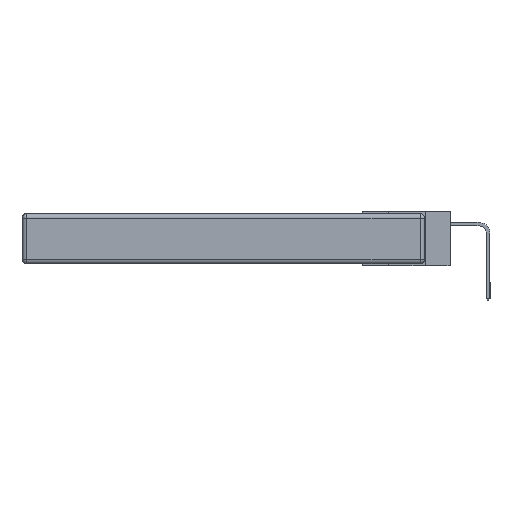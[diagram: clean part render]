
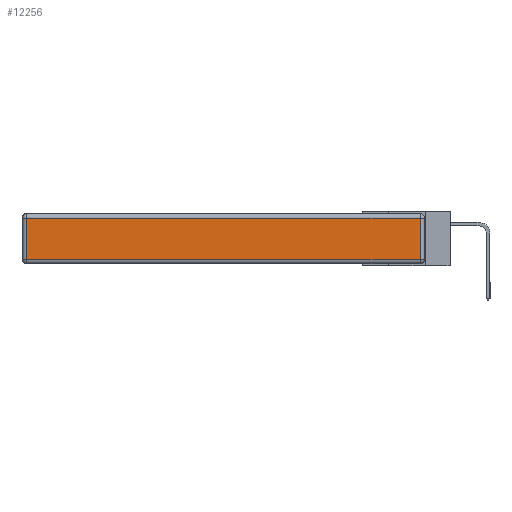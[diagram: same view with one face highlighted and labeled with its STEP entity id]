
A CAD part, left-side view. The second image highlights one B-rep face of the part: STEP entity #12256.
In plain terms, the highlighted planar face has unit normal (-1, 0, 0).
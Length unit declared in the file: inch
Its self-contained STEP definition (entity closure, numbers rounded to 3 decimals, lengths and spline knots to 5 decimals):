
#117 = ORIENTED_EDGE ( 'NONE', *, *, #951, .T. ) ;
#170 = LINE ( 'NONE', #16541, #20174 ) ;
#203 = ORIENTED_EDGE ( 'NONE', *, *, #2006, .T. ) ;
#951 = EDGE_CURVE ( 'NONE', #13777, #20376, #170, .T. ) ;
#1790 = DIRECTION ( 'NONE',  ( 0., -1., 0. ) ) ;
#2006 = EDGE_CURVE ( 'NONE', #2697, #15702, #15984, .T. ) ;
#2697 = VERTEX_POINT ( 'NONE', #5781 ) ;
#3140 = CARTESIAN_POINT ( 'NONE',  ( 0., 0., -0.343 ) ) ;
#4662 = PLANE ( 'NONE',  #16591 ) ;
#5092 = EDGE_LOOP ( 'NONE', ( #7054, #203, #15507, #117 ) ) ;
#5781 = CARTESIAN_POINT ( 'NONE',  ( 0., 0.03, -0.313 ) ) ;
#6127 = CARTESIAN_POINT ( 'NONE',  ( 0., 0.03, -0.343 ) ) ;
#6984 = DIRECTION ( 'NONE',  ( 0., 0., -1. ) ) ;
#7054 = ORIENTED_EDGE ( 'NONE', *, *, #9627, .T. ) ;
#7376 = EDGE_CURVE ( 'NONE', #15702, #13777, #20122, .T. ) ;
#7848 = DIRECTION ( 'NONE',  ( 0., 0., 1. ) ) ;
#9627 = EDGE_CURVE ( 'NONE', #20376, #2697, #16001, .T. ) ;
#9669 = DIRECTION ( 'NONE',  ( -1., 0., 0. ) ) ;
#10527 = DIRECTION ( 'NONE',  ( 0., 1., 0. ) ) ;
#11320 = CARTESIAN_POINT ( 'NONE',  ( 0., 2.72, -0.313 ) ) ;
#11390 = FACE_OUTER_BOUND ( 'NONE', #5092, .T. ) ;
#11448 = CARTESIAN_POINT ( 'NONE',  ( 0., 0.03, -0.03 ) ) ;
#11622 = VECTOR ( 'NONE', #10527, 39.37008 ) ;
#11789 = VECTOR ( 'NONE', #1790, 39.37008 ) ;
#12256 = ADVANCED_FACE ( 'NONE', ( #11390 ), #4662, .T. ) ;
#12723 = DIRECTION ( 'NONE',  ( 0., 0., 1. ) ) ;
#13777 = VERTEX_POINT ( 'NONE', #15930 ) ;
#13913 = CARTESIAN_POINT ( 'NONE',  ( 0., 2.75, -0.03 ) ) ;
#13992 = VECTOR ( 'NONE', #12723, 39.37008 ) ;
#15507 = ORIENTED_EDGE ( 'NONE', *, *, #7376, .T. ) ;
#15702 = VERTEX_POINT ( 'NONE', #11448 ) ;
#15930 = CARTESIAN_POINT ( 'NONE',  ( 0., 2.72, -0.03 ) ) ;
#15984 = LINE ( 'NONE', #6127, #13992 ) ;
#16001 = LINE ( 'NONE', #19513, #11789 ) ;
#16541 = CARTESIAN_POINT ( 'NONE',  ( 0., 2.72, -0.343 ) ) ;
#16591 = AXIS2_PLACEMENT_3D ( 'NONE', #3140, #9669, #7848 ) ;
#19513 = CARTESIAN_POINT ( 'NONE',  ( 0., 0., -0.313 ) ) ;
#20122 = LINE ( 'NONE', #13913, #11622 ) ;
#20174 = VECTOR ( 'NONE', #6984, 39.37008 ) ;
#20376 = VERTEX_POINT ( 'NONE', #11320 ) ;
